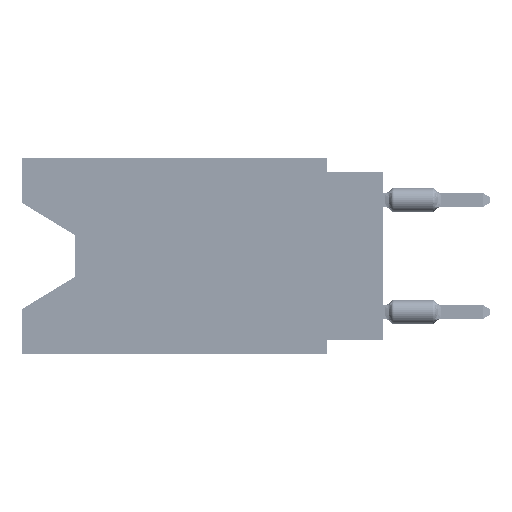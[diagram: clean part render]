
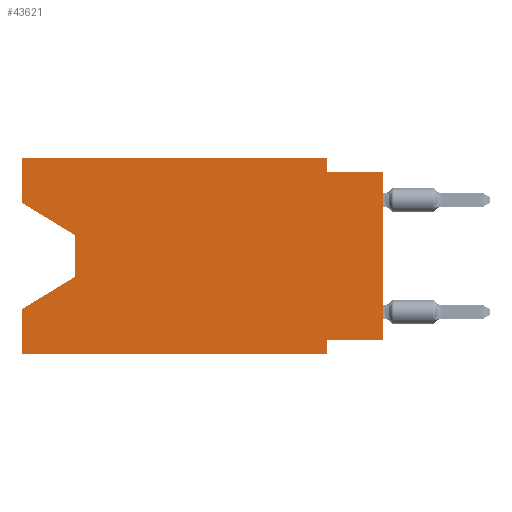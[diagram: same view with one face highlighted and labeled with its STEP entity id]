
A CAD part, left-side view. The second image highlights one B-rep face of the part: STEP entity #43621.
In plain terms, the highlighted planar face has unit normal (-1, 0, 0).
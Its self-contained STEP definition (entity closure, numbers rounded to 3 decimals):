
#505 = CARTESIAN_POINT ( 'NONE',  ( 0., 2.54, -8.89 ) ) ;
#1677 = CARTESIAN_POINT ( 'NONE',  ( 0., 16.383, 0. ) ) ;
#1990 = CARTESIAN_POINT ( 'NONE',  ( 0., 0., -0.635 ) ) ;
#2519 = LINE ( 'NONE', #7008, #8806 ) ;
#2790 = CARTESIAN_POINT ( 'NONE',  ( 0., 16.383, 0. ) ) ;
#2981 = VERTEX_POINT ( 'NONE', #59268 ) ;
#3815 = VERTEX_POINT ( 'NONE', #37406 ) ;
#4641 = DIRECTION ( 'NONE',  ( 0., 0., -1. ) ) ;
#5113 = VERTEX_POINT ( 'NONE', #505 ) ;
#5286 = DIRECTION ( 'NONE',  ( 0., -0.855, -0.519 ) ) ;
#6151 = CARTESIAN_POINT ( 'NONE',  ( 0., 0., -8.255 ) ) ;
#6463 = LINE ( 'NONE', #1677, #48918 ) ;
#6635 = LINE ( 'NONE', #2790, #36885 ) ;
#7008 = CARTESIAN_POINT ( 'NONE',  ( 0., 0., 0. ) ) ;
#7016 = VECTOR ( 'NONE', #28082, 1000. ) ;
#7645 = DIRECTION ( 'NONE',  ( 0., 0., 1. ) ) ;
#8166 = LINE ( 'NONE', #57196, #7016 ) ;
#8672 = DIRECTION ( 'NONE',  ( 0., 0., -1. ) ) ;
#8806 = VECTOR ( 'NONE', #7645, 1000. ) ;
#9600 = VERTEX_POINT ( 'NONE', #17740 ) ;
#10419 = LINE ( 'NONE', #10738, #61631 ) ;
#10738 = CARTESIAN_POINT ( 'NONE',  ( 0., 16.383, -2.038 ) ) ;
#14041 = VERTEX_POINT ( 'NONE', #6151 ) ;
#14145 = VECTOR ( 'NONE', #22146, 1000. ) ;
#14875 = DIRECTION ( 'NONE',  ( 0., 0.855, -0.519 ) ) ;
#16077 = LINE ( 'NONE', #34345, #45394 ) ;
#16298 = ORIENTED_EDGE ( 'NONE', *, *, #34395, .T. ) ;
#16491 = ORIENTED_EDGE ( 'NONE', *, *, #26051, .F. ) ;
#16544 = DIRECTION ( 'NONE',  ( 0., 0., 1. ) ) ;
#17740 = CARTESIAN_POINT ( 'NONE',  ( 0., 16.383, -6.852 ) ) ;
#18013 = LINE ( 'NONE', #37547, #21450 ) ;
#21244 = DIRECTION ( 'NONE',  ( 0., 0., 1. ) ) ;
#21450 = VECTOR ( 'NONE', #8672, 1000. ) ;
#22146 = DIRECTION ( 'NONE',  ( 0., 1., 0. ) ) ;
#22636 = EDGE_CURVE ( 'NONE', #44654, #9600, #6463, .T. ) ;
#24375 = CARTESIAN_POINT ( 'NONE',  ( 0., 16.383, 0. ) ) ;
#25408 = EDGE_CURVE ( 'NONE', #39797, #3815, #16077, .T. ) ;
#26051 = EDGE_CURVE ( 'NONE', #35009, #44661, #31938, .T. ) ;
#26340 = CARTESIAN_POINT ( 'NONE',  ( 0., 0., -8.255 ) ) ;
#28082 = DIRECTION ( 'NONE',  ( 0., -1., 0. ) ) ;
#29214 = VERTEX_POINT ( 'NONE', #24375 ) ;
#29406 = EDGE_CURVE ( 'NONE', #14041, #44661, #2519, .T. ) ;
#31938 = LINE ( 'NONE', #51454, #46495 ) ;
#32011 = AXIS2_PLACEMENT_3D ( 'NONE', #53026, #48541, #4641 ) ;
#33236 = EDGE_CURVE ( 'NONE', #29214, #2981, #6635, .T. ) ;
#33827 = FACE_OUTER_BOUND ( 'NONE', #55212, .T. ) ;
#34147 = PLANE ( 'NONE',  #32011 ) ;
#34345 = CARTESIAN_POINT ( 'NONE',  ( 0., 13.97, -3.505 ) ) ;
#34395 = EDGE_CURVE ( 'NONE', #3815, #9600, #56219, .T. ) ;
#35009 = VERTEX_POINT ( 'NONE', #50552 ) ;
#35510 = DIRECTION ( 'NONE',  ( 0., 0., -1. ) ) ;
#36454 = DIRECTION ( 'NONE',  ( 0., -1., 0. ) ) ;
#36760 = CARTESIAN_POINT ( 'NONE',  ( 0., 2.54, -8.89 ) ) ;
#36885 = VECTOR ( 'NONE', #36454, 1000. ) ;
#37406 = CARTESIAN_POINT ( 'NONE',  ( 0., 13.97, -5.385 ) ) ;
#37547 = CARTESIAN_POINT ( 'NONE',  ( 0., 2.54, 0. ) ) ;
#37978 = ORIENTED_EDGE ( 'NONE', *, *, #25408, .T. ) ;
#39057 = CARTESIAN_POINT ( 'NONE',  ( 0., 16.383, 0. ) ) ;
#39797 = VERTEX_POINT ( 'NONE', #40909 ) ;
#40909 = CARTESIAN_POINT ( 'NONE',  ( 0., 13.97, -3.505 ) ) ;
#40940 = LINE ( 'NONE', #36760, #41369 ) ;
#41369 = VECTOR ( 'NONE', #35510, 1000. ) ;
#41850 = DIRECTION ( 'NONE',  ( 0., -1., 0. ) ) ;
#42021 = CARTESIAN_POINT ( 'NONE',  ( 0., 16.383, -8.89 ) ) ;
#42452 = ORIENTED_EDGE ( 'NONE', *, *, #49898, .F. ) ;
#42945 = ORIENTED_EDGE ( 'NONE', *, *, #33236, .F. ) ;
#43621 = ADVANCED_FACE ( 'NONE', ( #33827 ), #34147, .F. ) ;
#43928 = DIRECTION ( 'NONE',  ( 0., 0., -1. ) ) ;
#44108 = VECTOR ( 'NONE', #14875, 1000. ) ;
#44211 = CARTESIAN_POINT ( 'NONE',  ( 0., 16.383, -2.038 ) ) ;
#44654 = VERTEX_POINT ( 'NONE', #42021 ) ;
#44661 = VERTEX_POINT ( 'NONE', #1990 ) ;
#44804 = VERTEX_POINT ( 'NONE', #44211 ) ;
#44898 = ORIENTED_EDGE ( 'NONE', *, *, #50828, .T. ) ;
#45394 = VECTOR ( 'NONE', #43928, 1000. ) ;
#45460 = EDGE_CURVE ( 'NONE', #45917, #5113, #40940, .T. ) ;
#45841 = ORIENTED_EDGE ( 'NONE', *, *, #51574, .T. ) ;
#45917 = VERTEX_POINT ( 'NONE', #50136 ) ;
#45974 = LINE ( 'NONE', #39057, #61528 ) ;
#46495 = VECTOR ( 'NONE', #41850, 1000. ) ;
#48541 = DIRECTION ( 'NONE',  ( 1., 0., 0. ) ) ;
#48918 = VECTOR ( 'NONE', #21244, 1000. ) ;
#49898 = EDGE_CURVE ( 'NONE', #14041, #45917, #60887, .T. ) ;
#50136 = CARTESIAN_POINT ( 'NONE',  ( 0., 2.54, -8.255 ) ) ;
#50552 = CARTESIAN_POINT ( 'NONE',  ( 0., 2.54, -0.635 ) ) ;
#50828 = EDGE_CURVE ( 'NONE', #44654, #5113, #8166, .T. ) ;
#51377 = ORIENTED_EDGE ( 'NONE', *, *, #52305, .F. ) ;
#51454 = CARTESIAN_POINT ( 'NONE',  ( 0., 0., -0.635 ) ) ;
#51574 = EDGE_CURVE ( 'NONE', #44804, #39797, #10419, .T. ) ;
#52305 = EDGE_CURVE ( 'NONE', #44804, #29214, #45974, .T. ) ;
#52755 = ORIENTED_EDGE ( 'NONE', *, *, #45460, .F. ) ;
#53026 = CARTESIAN_POINT ( 'NONE',  ( 0., 16.383, 0. ) ) ;
#53297 = CARTESIAN_POINT ( 'NONE',  ( 0., 13.97, -5.385 ) ) ;
#54937 = ORIENTED_EDGE ( 'NONE', *, *, #22636, .F. ) ;
#55212 = EDGE_LOOP ( 'NONE', ( #45841, #37978, #16298, #54937, #44898, #52755, #42452, #61400, #16491, #60984, #42945, #51377 ) ) ;
#56219 = LINE ( 'NONE', #53297, #44108 ) ;
#57196 = CARTESIAN_POINT ( 'NONE',  ( 0., 16.383, -8.89 ) ) ;
#59268 = CARTESIAN_POINT ( 'NONE',  ( 0., 2.54, 0. ) ) ;
#60887 = LINE ( 'NONE', #26340, #14145 ) ;
#60984 = ORIENTED_EDGE ( 'NONE', *, *, #63180, .F. ) ;
#61400 = ORIENTED_EDGE ( 'NONE', *, *, #29406, .T. ) ;
#61528 = VECTOR ( 'NONE', #16544, 1000. ) ;
#61631 = VECTOR ( 'NONE', #5286, 1000. ) ;
#63180 = EDGE_CURVE ( 'NONE', #2981, #35009, #18013, .T. ) ;
